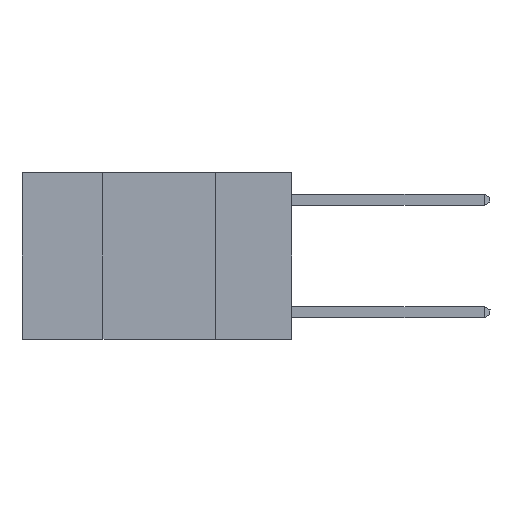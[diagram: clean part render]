
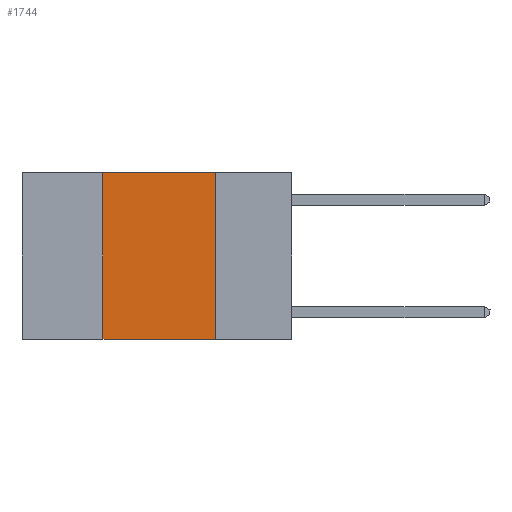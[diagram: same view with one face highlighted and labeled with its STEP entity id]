
A CAD part, left-side view. The second image highlights one B-rep face of the part: STEP entity #1744.
In plain terms, the highlighted planar face has unit normal (-1, 0, 0).
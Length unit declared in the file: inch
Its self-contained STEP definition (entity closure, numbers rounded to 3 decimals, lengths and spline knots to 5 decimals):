
#300 = LINE ( 'NONE', #26573, #25089 ) ;
#561 = FACE_OUTER_BOUND ( 'NONE', #24977, .T. ) ;
#1744 = ADVANCED_FACE ( 'NONE', ( #561 ), #4372, .F. ) ;
#2431 = EDGE_CURVE ( 'NONE', #10406, #5612, #300, .T. ) ;
#2552 = CARTESIAN_POINT ( 'NONE',  ( 0., 0.17, 0. ) ) ;
#2748 = CARTESIAN_POINT ( 'NONE',  ( 0., 0.42, 0. ) ) ;
#4372 = PLANE ( 'NONE',  #22970 ) ;
#4495 = EDGE_CURVE ( 'NONE', #23682, #4647, #25312, .T. ) ;
#4647 = VERTEX_POINT ( 'NONE', #20999 ) ;
#4706 = CARTESIAN_POINT ( 'NONE',  ( 0., 0.17, 0. ) ) ;
#5287 = CARTESIAN_POINT ( 'NONE',  ( 0., 0.42, 0. ) ) ;
#5612 = VERTEX_POINT ( 'NONE', #2552 ) ;
#5633 = ORIENTED_EDGE ( 'NONE', *, *, #2431, .F. ) ;
#6300 = VECTOR ( 'NONE', #10884, 39.37008 ) ;
#7762 = DIRECTION ( 'NONE',  ( 0., 0., 1. ) ) ;
#8421 = CARTESIAN_POINT ( 'NONE',  ( 0., 0.6, -0.37 ) ) ;
#9304 = DIRECTION ( 'NONE',  ( 0., 0., -1. ) ) ;
#10406 = VERTEX_POINT ( 'NONE', #2748 ) ;
#10884 = DIRECTION ( 'NONE',  ( 0., -1., 0. ) ) ;
#12175 = DIRECTION ( 'NONE',  ( 0., 0., -1. ) ) ;
#12486 = DIRECTION ( 'NONE',  ( 0., -1., 0. ) ) ;
#15890 = EDGE_CURVE ( 'NONE', #23682, #10406, #26181, .T. ) ;
#16557 = ORIENTED_EDGE ( 'NONE', *, *, #26868, .F. ) ;
#19766 = VECTOR ( 'NONE', #12175, 39.37008 ) ;
#20117 = ORIENTED_EDGE ( 'NONE', *, *, #4495, .T. ) ;
#20541 = LINE ( 'NONE', #4706, #19766 ) ;
#20999 = CARTESIAN_POINT ( 'NONE',  ( 0., 0.17, -0.37 ) ) ;
#21220 = CARTESIAN_POINT ( 'NONE',  ( 0., 0.6, 0. ) ) ;
#22970 = AXIS2_PLACEMENT_3D ( 'NONE', #21220, #23515, #9304 ) ;
#23515 = DIRECTION ( 'NONE',  ( 1., 0., 0. ) ) ;
#23682 = VERTEX_POINT ( 'NONE', #23853 ) ;
#23853 = CARTESIAN_POINT ( 'NONE',  ( 0., 0.42, -0.37 ) ) ;
#24977 = EDGE_LOOP ( 'NONE', ( #16557, #5633, #25545, #20117 ) ) ;
#25089 = VECTOR ( 'NONE', #12486, 39.37008 ) ;
#25312 = LINE ( 'NONE', #8421, #6300 ) ;
#25468 = VECTOR ( 'NONE', #7762, 39.37008 ) ;
#25545 = ORIENTED_EDGE ( 'NONE', *, *, #15890, .F. ) ;
#26181 = LINE ( 'NONE', #5287, #25468 ) ;
#26573 = CARTESIAN_POINT ( 'NONE',  ( 0., 0.6, 0. ) ) ;
#26868 = EDGE_CURVE ( 'NONE', #5612, #4647, #20541, .T. ) ;
